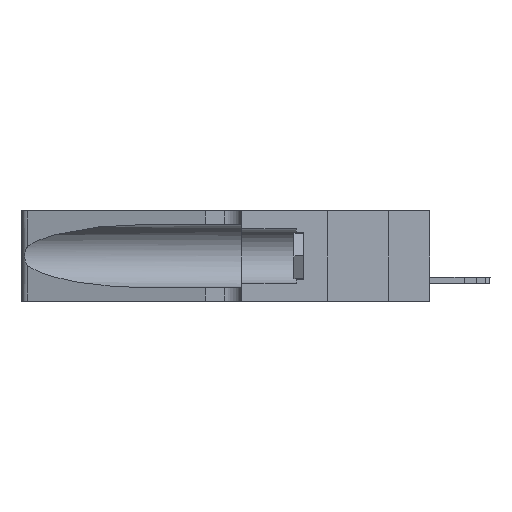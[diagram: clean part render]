
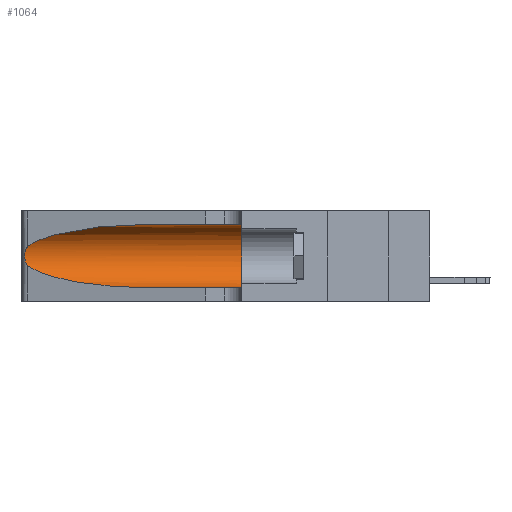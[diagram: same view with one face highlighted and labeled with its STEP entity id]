
A CAD part, left-side view. The second image highlights one B-rep face of the part: STEP entity #1064.
In plain terms, the highlighted cylindrical face has radius 3.308 mm (diameter 6.617 mm), a partial arc.
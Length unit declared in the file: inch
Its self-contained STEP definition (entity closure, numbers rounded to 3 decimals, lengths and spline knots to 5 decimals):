
#45 = CARTESIAN_POINT ( 'NONE',  ( 0.1305, 0.35, 0.31525 ) ) ;
#294 = VERTEX_POINT ( 'NONE', #12999 ) ;
#555 = ORIENTED_EDGE ( 'NONE', *, *, #17916, .T. ) ;
#1060 = VERTEX_POINT ( 'NONE', #4296 ) ;
#1064 = ADVANCED_FACE ( 'NONE', ( #13499 ), #12347, .F. ) ;
#1145 = CARTESIAN_POINT ( 'NONE',  ( 0.25487, 1.22718, 0.14631 ) ) ;
#2734 = CARTESIAN_POINT ( 'NONE',  ( 0.26075, 1.23896, 0.19203 ) ) ;
#3144 = CARTESIAN_POINT ( 'NONE',  ( 0.1305, 1.61858, 0.05475 ) ) ;
#4147 = CARTESIAN_POINT ( 'NONE',  ( 0.25854, 1.2359, 0.20912 ) ) ;
#4282 = CARTESIAN_POINT ( 'NONE',  ( 0.2373, 1.15595, 0.08982 ) ) ;
#4296 = CARTESIAN_POINT ( 'NONE',  ( 0.1305, 0.72297, 0.31525 ) ) ;
#4945 = VERTEX_POINT ( 'NONE', #15312 ) ;
#5012 = CARTESIAN_POINT ( 'NONE',  ( 0.1305, 0.72297, 0.31525 ) ) ;
#5104 = VECTOR ( 'NONE', #6208, 39.37008 ) ;
#5666 = CARTESIAN_POINT ( 'NONE',  ( 0.26017, 1.23833, 0.17102 ) ) ;
#5897 = CARTESIAN_POINT ( 'NONE',  ( 0.1305, 0.35, 0.185 ) ) ;
#5957 = CIRCLE ( 'NONE', #8869, 0.13025 ) ;
#5972 = ORIENTED_EDGE ( 'NONE', *, *, #10838, .T. ) ;
#6025 = EDGE_CURVE ( 'NONE', #11506, #294, #13803, .T. ) ;
#6208 = DIRECTION ( 'NONE',  ( 0., -1., 0. ) ) ;
#6547 = ORIENTED_EDGE ( 'NONE', *, *, #8116, .F. ) ;
#7016 = EDGE_LOOP ( 'NONE', ( #555, #5972, #14525, #15410, #16162, #6547 ) ) ;
#7102 = CARTESIAN_POINT ( 'NONE',  ( 0.25787, 1.23484, 0.2124 ) ) ;
#7240 = CARTESIAN_POINT ( 'NONE',  ( 0.25555, 1.22994, 0.2215 ) ) ;
#7326 = DIRECTION ( 'NONE',  ( 0., -1., 0. ) ) ;
#8116 = EDGE_CURVE ( 'NONE', #1060, #10059, #14700, .T. ) ;
#8618 = CARTESIAN_POINT ( 'NONE',  ( 0.25555, 1.22993, 0.14849 ) ) ;
#8626 = CARTESIAN_POINT ( 'NONE',  ( 0.18966, 0.96281, 0.05475 ) ) ;
#8869 = AXIS2_PLACEMENT_3D ( 'NONE', #5897, #19520, #19399 ) ;
#8881 = CARTESIAN_POINT ( 'NONE',  ( 0.26075, 1.23896, 0.178 ) ) ;
#9662 = VERTEX_POINT ( 'NONE', #11286 ) ;
#10059 = VERTEX_POINT ( 'NONE', #45 ) ;
#10838 = EDGE_CURVE ( 'NONE', #9662, #4945, #12566, .T. ) ;
#11286 = CARTESIAN_POINT ( 'NONE',  ( 0.25487, 1.22718, 0.22369 ) ) ;
#11492 =( BOUNDED_CURVE ( )  B_SPLINE_CURVE ( 3, ( #14703, #4282, #8626, #13157 ),
 .UNSPECIFIED., .F., .T. ) 
 B_SPLINE_CURVE_WITH_KNOTS ( ( 4, 4 ),
 ( 3.44316, 4.71239 ),
 .UNSPECIFIED. ) 
 CURVE ( )  GEOMETRIC_REPRESENTATION_ITEM ( )  RATIONAL_B_SPLINE_CURVE ( ( 1., 0.87, 0.87, 1. ) ) 
 REPRESENTATION_ITEM ( '' )  );
#11506 = VERTEX_POINT ( 'NONE', #17280 ) ;
#12143 = AXIS2_PLACEMENT_3D ( 'NONE', #13294, #7326, #17794 ) ;
#12347 = CYLINDRICAL_SURFACE ( 'NONE', #12143, 0.13025 ) ;
#12566 = B_SPLINE_CURVE_WITH_KNOTS ( 'NONE', 3,
 ( #14691, #7240, #19485, #7102, #4147, #19427, #2734, #8881, #5666, #17837, #14820, #13208, #8618, #1145 ),
 .UNSPECIFIED., .F., .F.,
 ( 4, 2, 2, 2, 2, 2, 4 ),
 ( 0., 0.00027, 0.00053, 0.00107, 0.0016, 0.00187, 0.00214 ),
 .UNSPECIFIED. ) ;
#12945 = CARTESIAN_POINT ( 'NONE',  ( 0.1305, 1.61858, 0.31525 ) ) ;
#12999 = CARTESIAN_POINT ( 'NONE',  ( 0.1305, 0.35, 0.05475 ) ) ;
#13157 = CARTESIAN_POINT ( 'NONE',  ( 0.1305, 0.72297, 0.05475 ) ) ;
#13208 = CARTESIAN_POINT ( 'NONE',  ( 0.25639, 1.23186, 0.15144 ) ) ;
#13294 = CARTESIAN_POINT ( 'NONE',  ( 0.1305, 1.61858, 0.185 ) ) ;
#13499 = FACE_OUTER_BOUND ( 'NONE', #7016, .T. ) ;
#13803 = LINE ( 'NONE', #3144, #5104 ) ;
#14151 = CARTESIAN_POINT ( 'NONE',  ( 0.25487, 1.22718, 0.22369 ) ) ;
#14229 = EDGE_CURVE ( 'NONE', #4945, #11506, #11492, .T. ) ;
#14525 = ORIENTED_EDGE ( 'NONE', *, *, #14229, .T. ) ;
#14691 = CARTESIAN_POINT ( 'NONE',  ( 0.25487, 1.22718, 0.22369 ) ) ;
#14700 = LINE ( 'NONE', #12945, #14926 ) ;
#14703 = CARTESIAN_POINT ( 'NONE',  ( 0.25487, 1.22718, 0.14631 ) ) ;
#14820 = CARTESIAN_POINT ( 'NONE',  ( 0.25789, 1.23486, 0.15765 ) ) ;
#14926 = VECTOR ( 'NONE', #18885, 39.37008 ) ;
#15312 = CARTESIAN_POINT ( 'NONE',  ( 0.25487, 1.22718, 0.14631 ) ) ;
#15383 = CARTESIAN_POINT ( 'NONE',  ( 0.18966, 0.96281, 0.31525 ) ) ;
#15410 = ORIENTED_EDGE ( 'NONE', *, *, #6025, .T. ) ;
#15697 = EDGE_CURVE ( 'NONE', #10059, #294, #5957, .T. ) ;
#16162 = ORIENTED_EDGE ( 'NONE', *, *, #15697, .F. ) ;
#17280 = CARTESIAN_POINT ( 'NONE',  ( 0.1305, 0.72297, 0.05475 ) ) ;
#17514 = CARTESIAN_POINT ( 'NONE',  ( 0.2373, 1.15595, 0.28018 ) ) ;
#17794 = DIRECTION ( 'NONE',  ( 0., 0., -1. ) ) ;
#17837 = CARTESIAN_POINT ( 'NONE',  ( 0.25856, 1.23593, 0.16098 ) ) ;
#17916 = EDGE_CURVE ( 'NONE', #1060, #9662, #18800, .T. ) ;
#18800 =( BOUNDED_CURVE ( )  B_SPLINE_CURVE ( 3, ( #5012, #15383, #17514, #14151 ),
 .UNSPECIFIED., .F., .T. ) 
 B_SPLINE_CURVE_WITH_KNOTS ( ( 4, 4 ),
 ( 1.5708, 2.84003 ),
 .UNSPECIFIED. ) 
 CURVE ( )  GEOMETRIC_REPRESENTATION_ITEM ( )  RATIONAL_B_SPLINE_CURVE ( ( 1., 0.87, 0.87, 1. ) ) 
 REPRESENTATION_ITEM ( '' )  );
#18885 = DIRECTION ( 'NONE',  ( 0., -1., 0. ) ) ;
#19399 = DIRECTION ( 'NONE',  ( 0., 0., 1. ) ) ;
#19427 = CARTESIAN_POINT ( 'NONE',  ( 0.26018, 1.23835, 0.19895 ) ) ;
#19485 = CARTESIAN_POINT ( 'NONE',  ( 0.25639, 1.23184, 0.21858 ) ) ;
#19520 = DIRECTION ( 'NONE',  ( 0., 1., 0. ) ) ;
